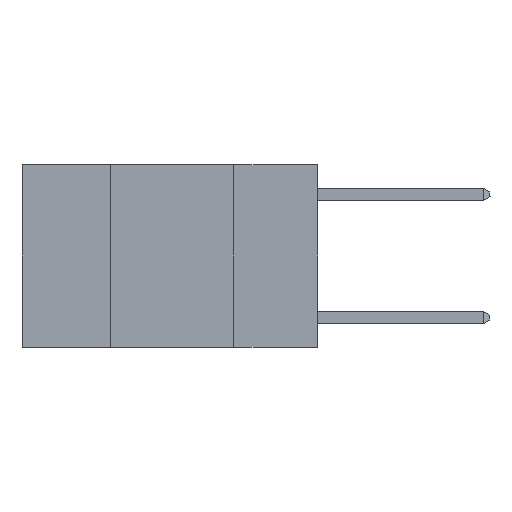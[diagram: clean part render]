
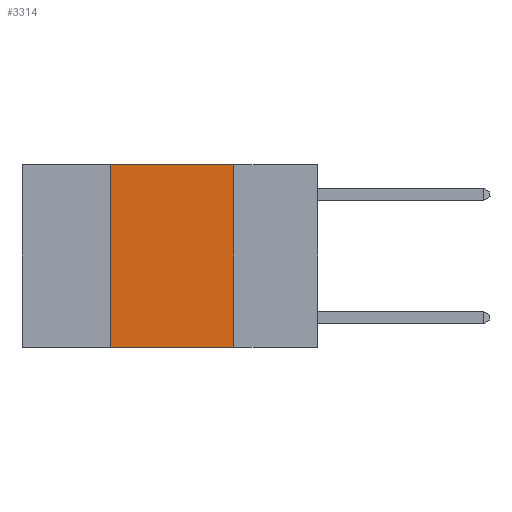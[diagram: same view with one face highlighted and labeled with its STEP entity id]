
A CAD part, left-side view. The second image highlights one B-rep face of the part: STEP entity #3314.
In plain terms, the highlighted planar face has unit normal (-1, 0, 0).
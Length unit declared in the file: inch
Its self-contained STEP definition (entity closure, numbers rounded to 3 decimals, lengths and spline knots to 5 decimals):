
#12 = ORIENTED_EDGE ( 'NONE', *, *, #9161, .F. ) ;
#38 = CARTESIAN_POINT ( 'NONE',  ( 0., 0.17, 0. ) ) ;
#214 = DIRECTION ( 'NONE',  ( 0., 0., 1. ) ) ;
#327 = PLANE ( 'NONE',  #3233 ) ;
#420 = DIRECTION ( 'NONE',  ( 0., 0., -1. ) ) ;
#575 = VERTEX_POINT ( 'NONE', #9450 ) ;
#730 = DIRECTION ( 'NONE',  ( 0., -1., 0. ) ) ;
#1020 = VERTEX_POINT ( 'NONE', #3653 ) ;
#1032 = CARTESIAN_POINT ( 'NONE',  ( 0., 0.42, 0. ) ) ;
#1055 = VECTOR ( 'NONE', #8315, 39.37008 ) ;
#1387 = EDGE_CURVE ( 'NONE', #6793, #1020, #6582, .T. ) ;
#1825 = ORIENTED_EDGE ( 'NONE', *, *, #1387, .F. ) ;
#2937 = ORIENTED_EDGE ( 'NONE', *, *, #6296, .T. ) ;
#3233 = AXIS2_PLACEMENT_3D ( 'NONE', #7382, #7015, #420 ) ;
#3314 = ADVANCED_FACE ( 'NONE', ( #3971 ), #327, .F. ) ;
#3591 = CARTESIAN_POINT ( 'NONE',  ( 0., 0.17, 0. ) ) ;
#3653 = CARTESIAN_POINT ( 'NONE',  ( 0., 0.17, -0.37 ) ) ;
#3795 = VECTOR ( 'NONE', #214, 39.37008 ) ;
#3971 = FACE_OUTER_BOUND ( 'NONE', #4743, .T. ) ;
#4743 = EDGE_LOOP ( 'NONE', ( #1825, #4911, #12, #2937 ) ) ;
#4836 = CARTESIAN_POINT ( 'NONE',  ( 0., 0.42, 0. ) ) ;
#4911 = ORIENTED_EDGE ( 'NONE', *, *, #6995, .F. ) ;
#5992 = LINE ( 'NONE', #8036, #6224 ) ;
#6224 = VECTOR ( 'NONE', #730, 39.37008 ) ;
#6296 = EDGE_CURVE ( 'NONE', #575, #1020, #5992, .T. ) ;
#6582 = LINE ( 'NONE', #38, #8797 ) ;
#6793 = VERTEX_POINT ( 'NONE', #3591 ) ;
#6902 = LINE ( 'NONE', #1032, #3795 ) ;
#6995 = EDGE_CURVE ( 'NONE', #7999, #6793, #9035, .T. ) ;
#7015 = DIRECTION ( 'NONE',  ( 1., 0., 0. ) ) ;
#7382 = CARTESIAN_POINT ( 'NONE',  ( 0., 0.6, 0. ) ) ;
#7999 = VERTEX_POINT ( 'NONE', #4836 ) ;
#8036 = CARTESIAN_POINT ( 'NONE',  ( 0., 0.6, -0.37 ) ) ;
#8315 = DIRECTION ( 'NONE',  ( 0., -1., 0. ) ) ;
#8797 = VECTOR ( 'NONE', #9406, 39.37008 ) ;
#8989 = CARTESIAN_POINT ( 'NONE',  ( 0., 0.6, 0. ) ) ;
#9035 = LINE ( 'NONE', #8989, #1055 ) ;
#9161 = EDGE_CURVE ( 'NONE', #575, #7999, #6902, .T. ) ;
#9406 = DIRECTION ( 'NONE',  ( 0., 0., -1. ) ) ;
#9450 = CARTESIAN_POINT ( 'NONE',  ( 0., 0.42, -0.37 ) ) ;
